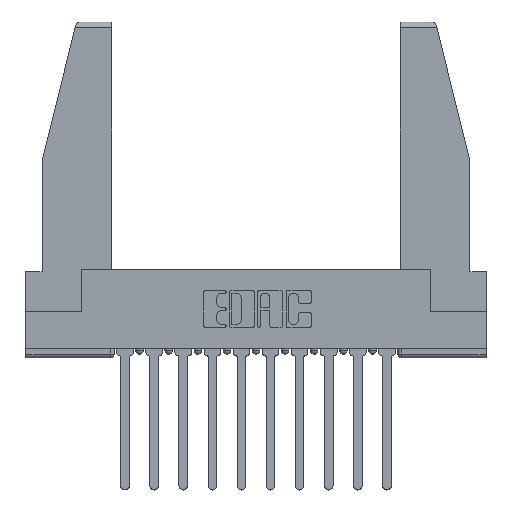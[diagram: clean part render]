
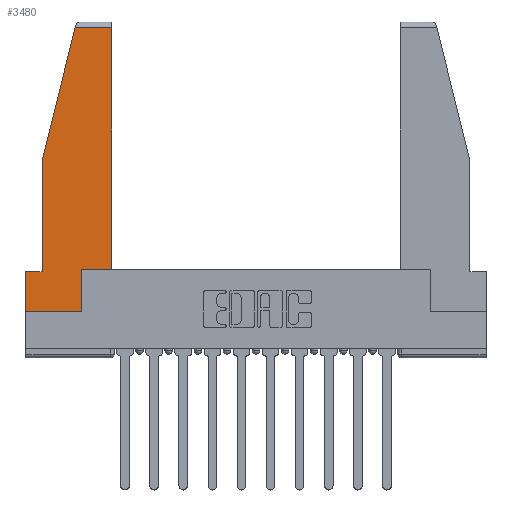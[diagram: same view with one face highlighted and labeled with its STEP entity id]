
A CAD part, top view. The second image highlights one B-rep face of the part: STEP entity #3480.
In plain terms, the highlighted planar face has unit normal (0, 0, 1).
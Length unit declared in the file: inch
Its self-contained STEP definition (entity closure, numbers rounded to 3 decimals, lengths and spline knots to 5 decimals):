
#206 = VERTEX_POINT ( 'NONE', #14698 ) ;
#495 = VECTOR ( 'NONE', #8982, 39.37008 ) ;
#603 = EDGE_CURVE ( 'NONE', #2696, #5738, #13828, .T. ) ;
#951 = VECTOR ( 'NONE', #12453, 39.37008 ) ;
#1052 = ORIENTED_EDGE ( 'NONE', *, *, #14575, .T. ) ;
#1093 = CARTESIAN_POINT ( 'NONE',  ( 0.271, 1.55, 0. ) ) ;
#1201 = VECTOR ( 'NONE', #13809, 39.37008 ) ;
#1497 = VERTEX_POINT ( 'NONE', #7984 ) ;
#1551 = LINE ( 'NONE', #14277, #13972 ) ;
#1675 = DIRECTION ( 'NONE',  ( -1., 0., 0. ) ) ;
#1806 = EDGE_CURVE ( 'NONE', #3645, #1497, #4261, .T. ) ;
#1984 = PLANE ( 'NONE',  #4028 ) ;
#2107 = DIRECTION ( 'NONE',  ( 0., -1., 0. ) ) ;
#2375 = EDGE_CURVE ( 'NONE', #3274, #13874, #11475, .T. ) ;
#2696 = VERTEX_POINT ( 'NONE', #3355 ) ;
#3127 = FACE_OUTER_BOUND ( 'NONE', #8625, .T. ) ;
#3274 = VERTEX_POINT ( 'NONE', #7548 ) ;
#3355 = CARTESIAN_POINT ( 'NONE',  ( 0.297, 0.223, 0. ) ) ;
#3480 = ADVANCED_FACE ( 'NONE', ( #3127 ), #1984, .T. ) ;
#3645 = VERTEX_POINT ( 'NONE', #7303 ) ;
#3850 = ORIENTED_EDGE ( 'NONE', *, *, #4536, .T. ) ;
#3900 = VERTEX_POINT ( 'NONE', #12538 ) ;
#4028 = AXIS2_PLACEMENT_3D ( 'NONE', #8966, #6777, #11357 ) ;
#4261 = LINE ( 'NONE', #10962, #10200 ) ;
#4468 = LINE ( 'NONE', #12386, #951 ) ;
#4536 = EDGE_CURVE ( 'NONE', #13874, #14080, #1551, .T. ) ;
#4624 = ORIENTED_EDGE ( 'NONE', *, *, #14206, .T. ) ;
#5071 = VECTOR ( 'NONE', #13383, 39.37008 ) ;
#5175 = CARTESIAN_POINT ( 'NONE',  ( 0.297, 0., 0. ) ) ;
#5529 = DIRECTION ( 'NONE',  ( 0., -1., 0. ) ) ;
#5738 = VERTEX_POINT ( 'NONE', #8389 ) ;
#6045 = VECTOR ( 'NONE', #2107, 39.37008 ) ;
#6675 = CARTESIAN_POINT ( 'NONE',  ( 0., 0.21, 0. ) ) ;
#6777 = DIRECTION ( 'NONE',  ( 0., 0., 1. ) ) ;
#6867 = LINE ( 'NONE', #1093, #1201 ) ;
#6980 = CARTESIAN_POINT ( 'NONE',  ( 0.086, 0.8, 0. ) ) ;
#7303 = CARTESIAN_POINT ( 'NONE',  ( 0.461, 1.52, 0. ) ) ;
#7548 = CARTESIAN_POINT ( 'NONE',  ( 0., 0.21, 0. ) ) ;
#7984 = CARTESIAN_POINT ( 'NONE',  ( 0.2636, 1.52, 0. ) ) ;
#8373 = VECTOR ( 'NONE', #5529, 39.37008 ) ;
#8389 = CARTESIAN_POINT ( 'NONE',  ( 0.461, 0.223, 0. ) ) ;
#8548 = VECTOR ( 'NONE', #12687, 39.37008 ) ;
#8625 = EDGE_LOOP ( 'NONE', ( #4624, #10796, #1052, #13276, #10792, #12214, #3850, #10991, #8683 ) ) ;
#8683 = ORIENTED_EDGE ( 'NONE', *, *, #603, .T. ) ;
#8966 = CARTESIAN_POINT ( 'NONE',  ( 0., 0., 0. ) ) ;
#8982 = DIRECTION ( 'NONE',  ( -1., 0., 0. ) ) ;
#9292 = CARTESIAN_POINT ( 'NONE',  ( 0.297, 0.223, 0. ) ) ;
#10200 = VECTOR ( 'NONE', #1675, 39.37008 ) ;
#10792 = ORIENTED_EDGE ( 'NONE', *, *, #14574, .T. ) ;
#10796 = ORIENTED_EDGE ( 'NONE', *, *, #1806, .T. ) ;
#10896 = LINE ( 'NONE', #12112, #5071 ) ;
#10962 = CARTESIAN_POINT ( 'NONE',  ( 0., 1.52, 0. ) ) ;
#10982 = DIRECTION ( 'NONE',  ( 1., 0., 0. ) ) ;
#10991 = ORIENTED_EDGE ( 'NONE', *, *, #13542, .T. ) ;
#11357 = DIRECTION ( 'NONE',  ( 1., 0., 0. ) ) ;
#11475 = LINE ( 'NONE', #6675, #8373 ) ;
#12112 = CARTESIAN_POINT ( 'NONE',  ( 0.297, 0., 0. ) ) ;
#12214 = ORIENTED_EDGE ( 'NONE', *, *, #2375, .T. ) ;
#12386 = CARTESIAN_POINT ( 'NONE',  ( 0.461, 0.223, 0. ) ) ;
#12453 = DIRECTION ( 'NONE',  ( 0., 1., 0. ) ) ;
#12538 = CARTESIAN_POINT ( 'NONE',  ( 0.086, 0.8, 0. ) ) ;
#12594 = LINE ( 'NONE', #14929, #495 ) ;
#12687 = DIRECTION ( 'NONE',  ( 1., 0., 0. ) ) ;
#12703 = LINE ( 'NONE', #6980, #6045 ) ;
#13276 = ORIENTED_EDGE ( 'NONE', *, *, #13763, .T. ) ;
#13383 = DIRECTION ( 'NONE',  ( 0., 1., 0. ) ) ;
#13542 = EDGE_CURVE ( 'NONE', #14080, #2696, #10896, .T. ) ;
#13763 = EDGE_CURVE ( 'NONE', #3900, #206, #12703, .T. ) ;
#13809 = DIRECTION ( 'NONE',  ( -0.239, -0.971, 0. ) ) ;
#13828 = LINE ( 'NONE', #9292, #8548 ) ;
#13874 = VERTEX_POINT ( 'NONE', #14149 ) ;
#13972 = VECTOR ( 'NONE', #10982, 39.37008 ) ;
#14080 = VERTEX_POINT ( 'NONE', #5175 ) ;
#14149 = CARTESIAN_POINT ( 'NONE',  ( 0., 0., 0. ) ) ;
#14206 = EDGE_CURVE ( 'NONE', #5738, #3645, #4468, .T. ) ;
#14277 = CARTESIAN_POINT ( 'NONE',  ( 0., 0., 0. ) ) ;
#14574 = EDGE_CURVE ( 'NONE', #206, #3274, #12594, .T. ) ;
#14575 = EDGE_CURVE ( 'NONE', #1497, #3900, #6867, .T. ) ;
#14698 = CARTESIAN_POINT ( 'NONE',  ( 0.086, 0.21, 0. ) ) ;
#14929 = CARTESIAN_POINT ( 'NONE',  ( 0., 0.21, 0. ) ) ;
